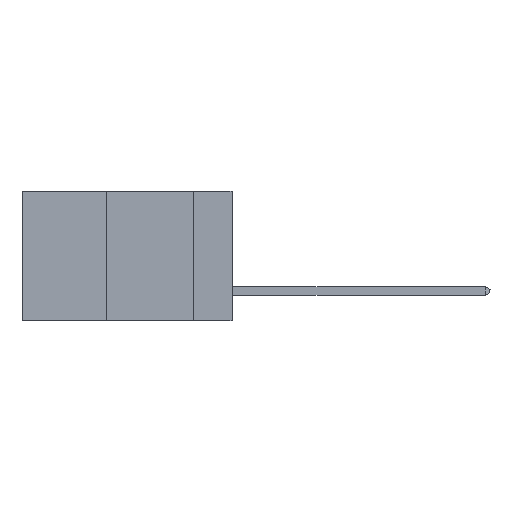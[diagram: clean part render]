
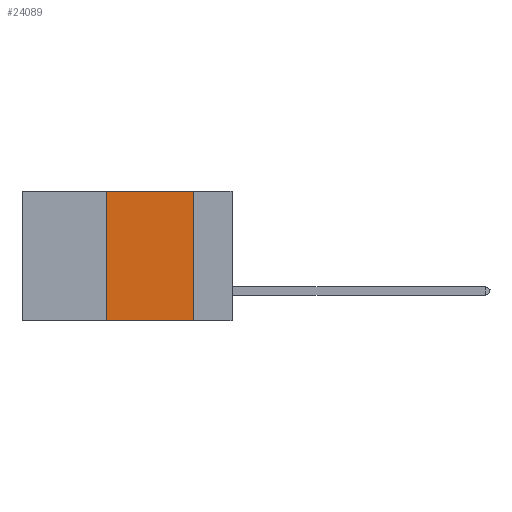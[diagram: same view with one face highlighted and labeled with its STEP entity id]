
A CAD part, left-side view. The second image highlights one B-rep face of the part: STEP entity #24089.
In plain terms, the highlighted planar face has unit normal (-1, 0, 0).
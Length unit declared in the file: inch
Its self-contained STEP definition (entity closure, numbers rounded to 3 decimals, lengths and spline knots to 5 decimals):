
#374 = DIRECTION ( 'NONE',  ( 0., 0., -1. ) ) ;
#829 = DIRECTION ( 'NONE',  ( 1., 0., 0. ) ) ;
#2033 = CARTESIAN_POINT ( 'NONE',  ( 0., 0.11, -0.37 ) ) ;
#2037 = DIRECTION ( 'NONE',  ( 0., 0., 1. ) ) ;
#3077 = LINE ( 'NONE', #3595, #32468 ) ;
#3595 = CARTESIAN_POINT ( 'NONE',  ( 0., 0.11, 0. ) ) ;
#4504 = VERTEX_POINT ( 'NONE', #2033 ) ;
#4657 = EDGE_LOOP ( 'NONE', ( #24816, #11659, #30301, #32229 ) ) ;
#5068 = DIRECTION ( 'NONE',  ( 0., -1., 0. ) ) ;
#5150 = VERTEX_POINT ( 'NONE', #30339 ) ;
#6254 = EDGE_CURVE ( 'NONE', #5150, #4504, #3077, .T. ) ;
#7485 = CARTESIAN_POINT ( 'NONE',  ( 0., 0.36, -0.37 ) ) ;
#8203 = FACE_OUTER_BOUND ( 'NONE', #4657, .T. ) ;
#8653 = VECTOR ( 'NONE', #2037, 39.37008 ) ;
#11057 = DIRECTION ( 'NONE',  ( 0., 0., -1. ) ) ;
#11543 = CARTESIAN_POINT ( 'NONE',  ( 0., 0.6, 0. ) ) ;
#11659 = ORIENTED_EDGE ( 'NONE', *, *, #31677, .F. ) ;
#15018 = AXIS2_PLACEMENT_3D ( 'NONE', #11543, #829, #11057 ) ;
#16103 = DIRECTION ( 'NONE',  ( 0., -1., 0. ) ) ;
#16781 = PLANE ( 'NONE',  #15018 ) ;
#17323 = LINE ( 'NONE', #34522, #32826 ) ;
#17429 = VECTOR ( 'NONE', #16103, 39.37008 ) ;
#18187 = CARTESIAN_POINT ( 'NONE',  ( 0., 0.36, 0. ) ) ;
#19134 = CARTESIAN_POINT ( 'NONE',  ( 0., 0.36, 0. ) ) ;
#22005 = LINE ( 'NONE', #29538, #17429 ) ;
#24089 = ADVANCED_FACE ( 'NONE', ( #8203 ), #16781, .F. ) ;
#24816 = ORIENTED_EDGE ( 'NONE', *, *, #6254, .F. ) ;
#24960 = VERTEX_POINT ( 'NONE', #7485 ) ;
#25622 = EDGE_CURVE ( 'NONE', #24960, #33632, #29667, .T. ) ;
#29538 = CARTESIAN_POINT ( 'NONE',  ( 0., 0.6, 0. ) ) ;
#29667 = LINE ( 'NONE', #18187, #8653 ) ;
#30301 = ORIENTED_EDGE ( 'NONE', *, *, #25622, .F. ) ;
#30339 = CARTESIAN_POINT ( 'NONE',  ( 0., 0.11, 0. ) ) ;
#31677 = EDGE_CURVE ( 'NONE', #33632, #5150, #22005, .T. ) ;
#32229 = ORIENTED_EDGE ( 'NONE', *, *, #32909, .T. ) ;
#32468 = VECTOR ( 'NONE', #374, 39.37008 ) ;
#32826 = VECTOR ( 'NONE', #5068, 39.37008 ) ;
#32909 = EDGE_CURVE ( 'NONE', #24960, #4504, #17323, .T. ) ;
#33632 = VERTEX_POINT ( 'NONE', #19134 ) ;
#34522 = CARTESIAN_POINT ( 'NONE',  ( 0., 0.6, -0.37 ) ) ;
